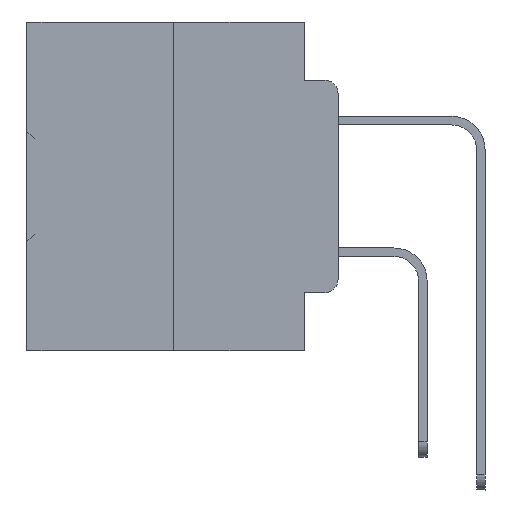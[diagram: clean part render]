
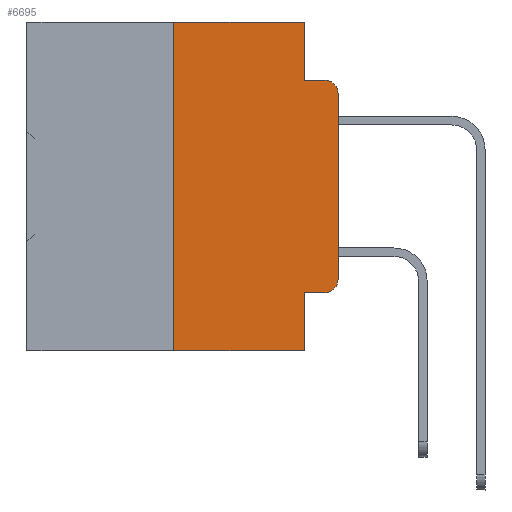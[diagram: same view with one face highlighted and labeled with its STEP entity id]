
A CAD part, left-side view. The second image highlights one B-rep face of the part: STEP entity #6695.
In plain terms, the highlighted planar face has unit normal (-1, 0, 0).
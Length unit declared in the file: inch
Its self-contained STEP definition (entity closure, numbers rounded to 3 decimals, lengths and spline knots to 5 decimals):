
#412 = VECTOR ( 'NONE', #4147, 39.37008 ) ;
#710 = EDGE_CURVE ( 'NONE', #25199, #38374, #36080, .T. ) ;
#841 = DIRECTION ( 'NONE',  ( 1., 0., 0. ) ) ;
#850 = EDGE_LOOP ( 'NONE', ( #6538, #7105, #39483, #19502, #20283, #5655, #15127, #33042, #25847, #22788 ) ) ;
#917 = CARTESIAN_POINT ( 'NONE',  ( 0., 0., 0. ) ) ;
#1157 = LINE ( 'NONE', #13612, #4989 ) ;
#2007 = DIRECTION ( 'NONE',  ( 0., 0., -1. ) ) ;
#2229 = VERTEX_POINT ( 'NONE', #33804 ) ;
#2823 = VERTEX_POINT ( 'NONE', #38238 ) ;
#3894 = CARTESIAN_POINT ( 'NONE',  ( 0., 0.473, 0. ) ) ;
#4147 = DIRECTION ( 'NONE',  ( 0., -1., 0. ) ) ;
#4595 = VECTOR ( 'NONE', #12686, 39.37008 ) ;
#4989 = VECTOR ( 'NONE', #19916, 39.37008 ) ;
#5055 = DIRECTION ( 'NONE',  ( -1., 0., 0. ) ) ;
#5135 = CARTESIAN_POINT ( 'NONE',  ( 0., 0.051, 0. ) ) ;
#5655 = ORIENTED_EDGE ( 'NONE', *, *, #9282, .F. ) ;
#5802 = CARTESIAN_POINT ( 'NONE',  ( 0., 0., -0.1085 ) ) ;
#6030 = DIRECTION ( 'NONE',  ( 0., -1., 0. ) ) ;
#6454 = EDGE_CURVE ( 'NONE', #18451, #2229, #39469, .T. ) ;
#6538 = ORIENTED_EDGE ( 'NONE', *, *, #33738, .T. ) ;
#6695 = ADVANCED_FACE ( 'NONE', ( #27994 ), #19189, .F. ) ;
#7105 = ORIENTED_EDGE ( 'NONE', *, *, #16505, .T. ) ;
#8075 = CARTESIAN_POINT ( 'NONE',  ( 0., 0.02, -0.3915 ) ) ;
#8807 = CARTESIAN_POINT ( 'NONE',  ( 0., 0.473, -0.5 ) ) ;
#9089 = CARTESIAN_POINT ( 'NONE',  ( 0., 0.051, -0.4115 ) ) ;
#9282 = EDGE_CURVE ( 'NONE', #18451, #23591, #31356, .T. ) ;
#11414 = VERTEX_POINT ( 'NONE', #5135 ) ;
#11886 = VERTEX_POINT ( 'NONE', #31077 ) ;
#12686 = DIRECTION ( 'NONE',  ( 0., 0., -1. ) ) ;
#12958 = CARTESIAN_POINT ( 'NONE',  ( 0., 0.25, 0. ) ) ;
#13051 = EDGE_CURVE ( 'NONE', #23591, #11414, #16212, .T. ) ;
#13612 = CARTESIAN_POINT ( 'NONE',  ( 0., 0.051, 0. ) ) ;
#14583 = DIRECTION ( 'NONE',  ( 0., -1., 0. ) ) ;
#15127 = ORIENTED_EDGE ( 'NONE', *, *, #6454, .T. ) ;
#15408 = CARTESIAN_POINT ( 'NONE',  ( 0., 0.25, 0. ) ) ;
#15819 = CARTESIAN_POINT ( 'NONE',  ( 0., 0.25, -0.5 ) ) ;
#16212 = LINE ( 'NONE', #19660, #412 ) ;
#16505 = EDGE_CURVE ( 'NONE', #24585, #2823, #29988, .T. ) ;
#16626 = LINE ( 'NONE', #917, #36696 ) ;
#18197 = EDGE_CURVE ( 'NONE', #33415, #2229, #1157, .T. ) ;
#18395 = DIRECTION ( 'NONE',  ( 0., -1., 0. ) ) ;
#18451 = VERTEX_POINT ( 'NONE', #15819 ) ;
#18486 = EDGE_CURVE ( 'NONE', #33415, #25199, #24600, .T. ) ;
#19189 = PLANE ( 'NONE',  #33931 ) ;
#19502 = ORIENTED_EDGE ( 'NONE', *, *, #29870, .F. ) ;
#19660 = CARTESIAN_POINT ( 'NONE',  ( 0., 0.473, 0. ) ) ;
#19916 = DIRECTION ( 'NONE',  ( 0., 0., -1. ) ) ;
#20283 = ORIENTED_EDGE ( 'NONE', *, *, #13051, .F. ) ;
#20390 = VECTOR ( 'NONE', #31957, 39.37008 ) ;
#20515 = DIRECTION ( 'NONE',  ( 0., 0., -1. ) ) ;
#22135 = VECTOR ( 'NONE', #18395, 39.37008 ) ;
#22275 = CARTESIAN_POINT ( 'NONE',  ( 0., 0.051, 0. ) ) ;
#22581 = VECTOR ( 'NONE', #6030, 39.37008 ) ;
#22788 = ORIENTED_EDGE ( 'NONE', *, *, #710, .T. ) ;
#23591 = VERTEX_POINT ( 'NONE', #15408 ) ;
#23746 = CARTESIAN_POINT ( 'NONE',  ( 0., 0.051, -0.0885 ) ) ;
#24585 = VERTEX_POINT ( 'NONE', #5802 ) ;
#24600 = LINE ( 'NONE', #9089, #22581 ) ;
#25199 = VERTEX_POINT ( 'NONE', #27996 ) ;
#25847 = ORIENTED_EDGE ( 'NONE', *, *, #18486, .T. ) ;
#26603 = LINE ( 'NONE', #23746, #32580 ) ;
#27994 = FACE_OUTER_BOUND ( 'NONE', #850, .T. ) ;
#27996 = CARTESIAN_POINT ( 'NONE',  ( 0., 0.02, -0.4115 ) ) ;
#28416 = LINE ( 'NONE', #22275, #4595 ) ;
#28429 = CARTESIAN_POINT ( 'NONE',  ( 0., 0., -0.3915 ) ) ;
#28690 = DIRECTION ( 'NONE',  ( 0., 0., 1. ) ) ;
#29870 = EDGE_CURVE ( 'NONE', #11414, #11886, #28416, .T. ) ;
#29988 = CIRCLE ( 'NONE', #33895, 0.02 ) ;
#30937 = EDGE_CURVE ( 'NONE', #11886, #2823, #26603, .T. ) ;
#31077 = CARTESIAN_POINT ( 'NONE',  ( 0., 0.051, -0.0885 ) ) ;
#31356 = LINE ( 'NONE', #12958, #20390 ) ;
#31957 = DIRECTION ( 'NONE',  ( 0., 0., 1. ) ) ;
#32401 = CARTESIAN_POINT ( 'NONE',  ( 0., 0.051, -0.4115 ) ) ;
#32580 = VECTOR ( 'NONE', #14583, 39.37008 ) ;
#32797 = DIRECTION ( 'NONE',  ( -1., 0., 0. ) ) ;
#33039 = CARTESIAN_POINT ( 'NONE',  ( 0., 0.02, -0.1085 ) ) ;
#33042 = ORIENTED_EDGE ( 'NONE', *, *, #18197, .F. ) ;
#33415 = VERTEX_POINT ( 'NONE', #32401 ) ;
#33738 = EDGE_CURVE ( 'NONE', #38374, #24585, #16626, .T. ) ;
#33804 = CARTESIAN_POINT ( 'NONE',  ( 0., 0.051, -0.5 ) ) ;
#33895 = AXIS2_PLACEMENT_3D ( 'NONE', #33039, #5055, #2007 ) ;
#33931 = AXIS2_PLACEMENT_3D ( 'NONE', #3894, #841, #38205 ) ;
#36080 = CIRCLE ( 'NONE', #40011, 0.02 ) ;
#36696 = VECTOR ( 'NONE', #28690, 39.37008 ) ;
#38205 = DIRECTION ( 'NONE',  ( 0., 0., -1. ) ) ;
#38238 = CARTESIAN_POINT ( 'NONE',  ( 0., 0.02, -0.0885 ) ) ;
#38374 = VERTEX_POINT ( 'NONE', #28429 ) ;
#39469 = LINE ( 'NONE', #8807, #22135 ) ;
#39483 = ORIENTED_EDGE ( 'NONE', *, *, #30937, .F. ) ;
#40011 = AXIS2_PLACEMENT_3D ( 'NONE', #8075, #32797, #20515 ) ;
